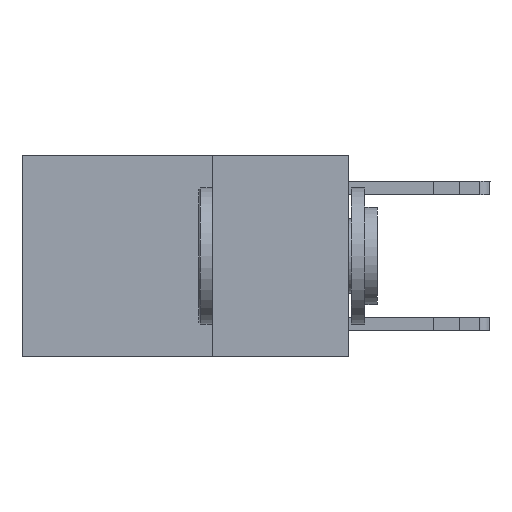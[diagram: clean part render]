
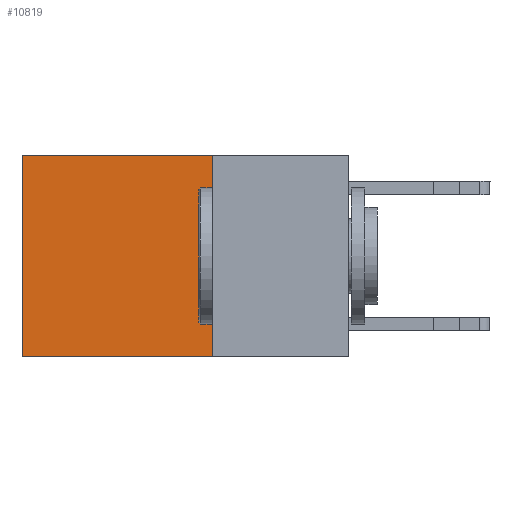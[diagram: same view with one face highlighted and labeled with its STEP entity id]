
A CAD part, left-side view. The second image highlights one B-rep face of the part: STEP entity #10819.
In plain terms, the highlighted planar face has unit normal (-1, 0, 0).
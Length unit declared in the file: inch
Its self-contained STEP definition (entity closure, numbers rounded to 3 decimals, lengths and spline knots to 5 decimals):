
#595 = VECTOR ( 'NONE', #18629, 39.37008 ) ;
#624 = ORIENTED_EDGE ( 'NONE', *, *, #8089, .F. ) ;
#645 = FACE_OUTER_BOUND ( 'NONE', #16005, .T. ) ;
#694 = CARTESIAN_POINT ( 'NONE',  ( 0.2625, 0.25, -0.37 ) ) ;
#1755 = VECTOR ( 'NONE', #16736, 39.37008 ) ;
#1795 = EDGE_CURVE ( 'NONE', #13091, #17994, #11466, .T. ) ;
#2269 = CARTESIAN_POINT ( 'NONE',  ( 0.2625, 0.25, 0. ) ) ;
#3117 = LINE ( 'NONE', #19003, #16511 ) ;
#4209 = DIRECTION ( 'NONE',  ( 1., 0., 0. ) ) ;
#6246 = VECTOR ( 'NONE', #16297, 39.37008 ) ;
#6665 = LINE ( 'NONE', #18746, #595 ) ;
#7466 = LINE ( 'NONE', #2269, #6246 ) ;
#7681 = PLANE ( 'NONE',  #17375 ) ;
#8089 = EDGE_CURVE ( 'NONE', #19481, #17994, #6665, .T. ) ;
#8648 = CARTESIAN_POINT ( 'NONE',  ( 0.2625, 0.25, 0. ) ) ;
#9182 = VERTEX_POINT ( 'NONE', #8648 ) ;
#9740 = CARTESIAN_POINT ( 'NONE',  ( 0.2625, 0.6, 0. ) ) ;
#10558 = CARTESIAN_POINT ( 'NONE',  ( 0.2625, 0.6, 0. ) ) ;
#10819 = ADVANCED_FACE ( 'NONE', ( #645 ), #7681, .F. ) ;
#11245 = DIRECTION ( 'NONE',  ( 0., 0., -1. ) ) ;
#11466 = LINE ( 'NONE', #9740, #1755 ) ;
#12958 = CARTESIAN_POINT ( 'NONE',  ( 0.2625, 0.25, 0. ) ) ;
#13091 = VERTEX_POINT ( 'NONE', #10558 ) ;
#14030 = EDGE_CURVE ( 'NONE', #9182, #19481, #3117, .T. ) ;
#14259 = ORIENTED_EDGE ( 'NONE', *, *, #20071, .T. ) ;
#14887 = ORIENTED_EDGE ( 'NONE', *, *, #1795, .T. ) ;
#16005 = EDGE_LOOP ( 'NONE', ( #14887, #624, #20367, #14259 ) ) ;
#16297 = DIRECTION ( 'NONE',  ( 0., 1., 0. ) ) ;
#16511 = VECTOR ( 'NONE', #19812, 39.37008 ) ;
#16736 = DIRECTION ( 'NONE',  ( 0., 0., -1. ) ) ;
#17375 = AXIS2_PLACEMENT_3D ( 'NONE', #12958, #4209, #11245 ) ;
#17994 = VERTEX_POINT ( 'NONE', #19353 ) ;
#18629 = DIRECTION ( 'NONE',  ( 0., 1., 0. ) ) ;
#18746 = CARTESIAN_POINT ( 'NONE',  ( 0.2625, 0.25, -0.37 ) ) ;
#19003 = CARTESIAN_POINT ( 'NONE',  ( 0.2625, 0.25, 0. ) ) ;
#19353 = CARTESIAN_POINT ( 'NONE',  ( 0.2625, 0.6, -0.37 ) ) ;
#19481 = VERTEX_POINT ( 'NONE', #694 ) ;
#19812 = DIRECTION ( 'NONE',  ( 0., 0., -1. ) ) ;
#20071 = EDGE_CURVE ( 'NONE', #9182, #13091, #7466, .T. ) ;
#20367 = ORIENTED_EDGE ( 'NONE', *, *, #14030, .F. ) ;
